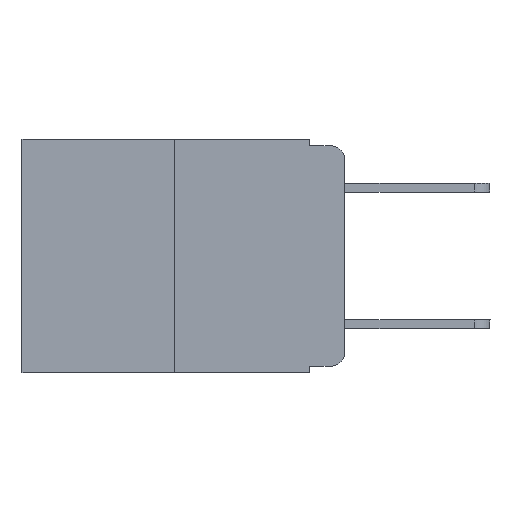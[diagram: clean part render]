
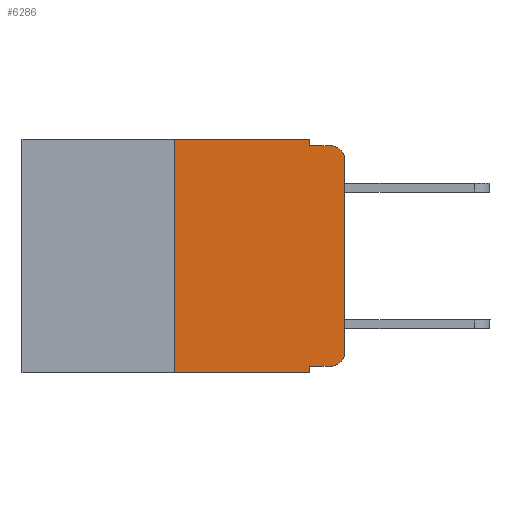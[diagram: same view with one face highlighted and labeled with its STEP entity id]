
A CAD part, left-side view. The second image highlights one B-rep face of the part: STEP entity #6286.
In plain terms, the highlighted planar face has unit normal (-1, 0, 0).
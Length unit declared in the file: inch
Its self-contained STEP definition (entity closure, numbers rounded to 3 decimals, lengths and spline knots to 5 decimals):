
#210 = DIRECTION ( 'NONE',  ( 0., 0., 1. ) ) ;
#573 = CARTESIAN_POINT ( 'NONE',  ( 0., 0., -0.313 ) ) ;
#847 = VERTEX_POINT ( 'NONE', #5477 ) ;
#1079 = CARTESIAN_POINT ( 'NONE',  ( 0., 0.25, -0.343 ) ) ;
#1510 = CARTESIAN_POINT ( 'NONE',  ( 0., 0.051, 0. ) ) ;
#1522 = CARTESIAN_POINT ( 'NONE',  ( 0., 0.473, -0.343 ) ) ;
#1860 = ORIENTED_EDGE ( 'NONE', *, *, #4339, .F. ) ;
#1932 = CARTESIAN_POINT ( 'NONE',  ( 0., 0., 0. ) ) ;
#1933 = CARTESIAN_POINT ( 'NONE',  ( 0., 0.02, -0.01 ) ) ;
#1952 = CARTESIAN_POINT ( 'NONE',  ( 0., 0.473, 0. ) ) ;
#2574 = VERTEX_POINT ( 'NONE', #14983 ) ;
#2973 = ORIENTED_EDGE ( 'NONE', *, *, #5917, .T. ) ;
#3031 = VECTOR ( 'NONE', #7593, 39.37008 ) ;
#3086 = CARTESIAN_POINT ( 'NONE',  ( 0., 0.051, -0.333 ) ) ;
#3447 = ORIENTED_EDGE ( 'NONE', *, *, #3874, .F. ) ;
#3579 = CARTESIAN_POINT ( 'NONE',  ( 0., 0.02, -0.03 ) ) ;
#3697 = LINE ( 'NONE', #14018, #13521 ) ;
#3874 = EDGE_CURVE ( 'NONE', #9820, #14637, #7907, .T. ) ;
#4339 = EDGE_CURVE ( 'NONE', #5747, #2574, #15195, .T. ) ;
#4440 = EDGE_CURVE ( 'NONE', #17456, #11948, #14180, .T. ) ;
#4576 = CARTESIAN_POINT ( 'NONE',  ( 0., 0., -0.03 ) ) ;
#4681 = VECTOR ( 'NONE', #9893, 39.37008 ) ;
#4779 = ORIENTED_EDGE ( 'NONE', *, *, #8158, .T. ) ;
#5002 = CARTESIAN_POINT ( 'NONE',  ( 0., 0.051, -0.01 ) ) ;
#5007 = ORIENTED_EDGE ( 'NONE', *, *, #6158, .T. ) ;
#5075 = DIRECTION ( 'NONE',  ( -1., 0., 0. ) ) ;
#5090 = DIRECTION ( 'NONE',  ( 1., 0., 0. ) ) ;
#5414 = ORIENTED_EDGE ( 'NONE', *, *, #11195, .F. ) ;
#5447 = DIRECTION ( 'NONE',  ( -1., 0., 0. ) ) ;
#5477 = CARTESIAN_POINT ( 'NONE',  ( 0., 0.02, -0.333 ) ) ;
#5747 = VERTEX_POINT ( 'NONE', #12100 ) ;
#5761 = VECTOR ( 'NONE', #18199, 39.37008 ) ;
#5846 = DIRECTION ( 'NONE',  ( 0., 0., -1. ) ) ;
#5859 = LINE ( 'NONE', #1932, #8540 ) ;
#5917 = EDGE_CURVE ( 'NONE', #9820, #2574, #12197, .T. ) ;
#6111 = VECTOR ( 'NONE', #9027, 39.37008 ) ;
#6158 = EDGE_CURVE ( 'NONE', #5747, #847, #13323, .T. ) ;
#6286 = ADVANCED_FACE ( 'NONE', ( #13975 ), #14931, .F. ) ;
#6629 = EDGE_CURVE ( 'NONE', #14637, #17456, #3697, .T. ) ;
#7568 = CARTESIAN_POINT ( 'NONE',  ( 0., 0.25, 0. ) ) ;
#7593 = DIRECTION ( 'NONE',  ( 0., -1., 0. ) ) ;
#7747 = LINE ( 'NONE', #18127, #5761 ) ;
#7907 = LINE ( 'NONE', #13044, #6111 ) ;
#7963 = DIRECTION ( 'NONE',  ( 0., 0., -1. ) ) ;
#8158 = EDGE_CURVE ( 'NONE', #8389, #16172, #15087, .T. ) ;
#8194 = EDGE_CURVE ( 'NONE', #847, #16699, #11694, .T. ) ;
#8374 = CARTESIAN_POINT ( 'NONE',  ( 0., 0.02, -0.313 ) ) ;
#8389 = VERTEX_POINT ( 'NONE', #4576 ) ;
#8540 = VECTOR ( 'NONE', #210, 39.37008 ) ;
#8754 = CARTESIAN_POINT ( 'NONE',  ( 0., 0.051, 0. ) ) ;
#9027 = DIRECTION ( 'NONE',  ( 0., 0., 1. ) ) ;
#9227 = CARTESIAN_POINT ( 'NONE',  ( 0., 0.051, 0. ) ) ;
#9820 = VERTEX_POINT ( 'NONE', #1079 ) ;
#9893 = DIRECTION ( 'NONE',  ( 0., 0., -1. ) ) ;
#10269 = ORIENTED_EDGE ( 'NONE', *, *, #4440, .F. ) ;
#10904 = ORIENTED_EDGE ( 'NONE', *, *, #8194, .T. ) ;
#11052 = AXIS2_PLACEMENT_3D ( 'NONE', #3579, #5075, #13574 ) ;
#11195 = EDGE_CURVE ( 'NONE', #11948, #16172, #7747, .T. ) ;
#11694 = CIRCLE ( 'NONE', #13223, 0.02 ) ;
#11948 = VERTEX_POINT ( 'NONE', #5002 ) ;
#12100 = CARTESIAN_POINT ( 'NONE',  ( 0., 0.051, -0.333 ) ) ;
#12197 = LINE ( 'NONE', #1522, #14922 ) ;
#13044 = CARTESIAN_POINT ( 'NONE',  ( 0., 0.25, 0. ) ) ;
#13223 = AXIS2_PLACEMENT_3D ( 'NONE', #8374, #5447, #14062 ) ;
#13323 = LINE ( 'NONE', #3086, #3031 ) ;
#13521 = VECTOR ( 'NONE', #16984, 39.37008 ) ;
#13574 = DIRECTION ( 'NONE',  ( 0., 0., -1. ) ) ;
#13614 = VECTOR ( 'NONE', #5846, 39.37008 ) ;
#13630 = EDGE_CURVE ( 'NONE', #16699, #8389, #5859, .T. ) ;
#13975 = FACE_OUTER_BOUND ( 'NONE', #14186, .T. ) ;
#14018 = CARTESIAN_POINT ( 'NONE',  ( 0., 0.473, 0. ) ) ;
#14062 = DIRECTION ( 'NONE',  ( 0., 0., -1. ) ) ;
#14180 = LINE ( 'NONE', #8754, #13614 ) ;
#14186 = EDGE_LOOP ( 'NONE', ( #17608, #4779, #5414, #10269, #16771, #3447, #2973, #1860, #5007, #10904 ) ) ;
#14637 = VERTEX_POINT ( 'NONE', #7568 ) ;
#14922 = VECTOR ( 'NONE', #17375, 39.37008 ) ;
#14931 = PLANE ( 'NONE',  #15984 ) ;
#14983 = CARTESIAN_POINT ( 'NONE',  ( 0., 0.051, -0.343 ) ) ;
#15087 = CIRCLE ( 'NONE', #11052, 0.02 ) ;
#15195 = LINE ( 'NONE', #1510, #4681 ) ;
#15984 = AXIS2_PLACEMENT_3D ( 'NONE', #1952, #5090, #7963 ) ;
#16172 = VERTEX_POINT ( 'NONE', #1933 ) ;
#16699 = VERTEX_POINT ( 'NONE', #573 ) ;
#16771 = ORIENTED_EDGE ( 'NONE', *, *, #6629, .F. ) ;
#16984 = DIRECTION ( 'NONE',  ( 0., -1., 0. ) ) ;
#17375 = DIRECTION ( 'NONE',  ( 0., -1., 0. ) ) ;
#17456 = VERTEX_POINT ( 'NONE', #9227 ) ;
#17608 = ORIENTED_EDGE ( 'NONE', *, *, #13630, .T. ) ;
#18127 = CARTESIAN_POINT ( 'NONE',  ( 0., 0.051, -0.01 ) ) ;
#18199 = DIRECTION ( 'NONE',  ( 0., -1., 0. ) ) ;
